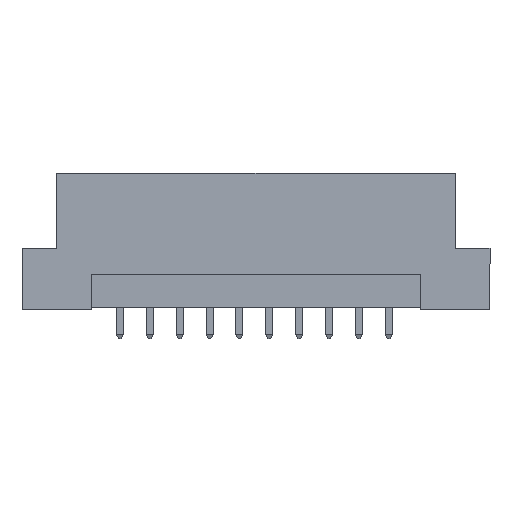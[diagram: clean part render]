
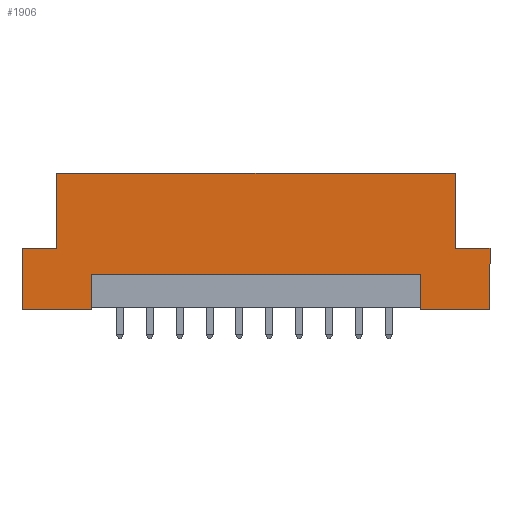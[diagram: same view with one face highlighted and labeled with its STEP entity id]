
A CAD part, front view. The second image highlights one B-rep face of the part: STEP entity #1906.
In plain terms, the highlighted planar face has unit normal (0, -1, 0).
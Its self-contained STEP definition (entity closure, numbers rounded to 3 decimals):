
#45 = VECTOR ( 'NONE', #1251, 1000. ) ;
#107 = ORIENTED_EDGE ( 'NONE', *, *, #4662, .T. ) ;
#114 = VERTEX_POINT ( 'NONE', #3270 ) ;
#131 = VECTOR ( 'NONE', #2270, 1000. ) ;
#250 = DIRECTION ( 'NONE',  ( 0., 0., 1. ) ) ;
#267 = EDGE_CURVE ( 'NONE', #1312, #3852, #4231, .T. ) ;
#430 = ORIENTED_EDGE ( 'NONE', *, *, #2387, .F. ) ;
#449 = CARTESIAN_POINT ( 'NONE',  ( -16.94, -4.3, 11.6 ) ) ;
#480 = VECTOR ( 'NONE', #901, 1000. ) ;
#522 = CARTESIAN_POINT ( 'NONE',  ( 19.9, -4.3, 0. ) ) ;
#525 = CARTESIAN_POINT ( 'NONE',  ( -14., -4.3, 3. ) ) ;
#536 = EDGE_CURVE ( 'NONE', #3905, #5048, #1664, .T. ) ;
#540 = LINE ( 'NONE', #2123, #2954 ) ;
#563 = ORIENTED_EDGE ( 'NONE', *, *, #3421, .F. ) ;
#606 = VECTOR ( 'NONE', #3008, 1000. ) ;
#608 = CARTESIAN_POINT ( 'NONE',  ( 19.9, -4.3, 11.6 ) ) ;
#617 = AXIS2_PLACEMENT_3D ( 'NONE', #4245, #5108, #2375 ) ;
#634 = CARTESIAN_POINT ( 'NONE',  ( -19.9, -4.3, 11.6 ) ) ;
#669 = EDGE_CURVE ( 'NONE', #3649, #3989, #4621, .T. ) ;
#682 = DIRECTION ( 'NONE',  ( 1., 0., 0. ) ) ;
#714 = CARTESIAN_POINT ( 'NONE',  ( -14., -4.3, 3. ) ) ;
#736 = VECTOR ( 'NONE', #1278, 1000. ) ;
#776 = VECTOR ( 'NONE', #1803, 1000. ) ;
#848 = VECTOR ( 'NONE', #2106, 1000. ) ;
#901 = DIRECTION ( 'NONE',  ( 0., 0., -1. ) ) ;
#1011 = LINE ( 'NONE', #1724, #776 ) ;
#1024 = VERTEX_POINT ( 'NONE', #3945 ) ;
#1050 = CARTESIAN_POINT ( 'NONE',  ( 19.9, -4.3, 0. ) ) ;
#1079 = DIRECTION ( 'NONE',  ( 1., 0., 0. ) ) ;
#1243 = EDGE_CURVE ( 'NONE', #3649, #114, #1011, .T. ) ;
#1251 = DIRECTION ( 'NONE',  ( 1., 0., 0. ) ) ;
#1278 = DIRECTION ( 'NONE',  ( 0., 0., -1. ) ) ;
#1280 = LINE ( 'NONE', #4136, #45 ) ;
#1312 = VERTEX_POINT ( 'NONE', #2902 ) ;
#1359 = VERTEX_POINT ( 'NONE', #525 ) ;
#1464 = CARTESIAN_POINT ( 'NONE',  ( -19.9, -4.3, 0. ) ) ;
#1664 = LINE ( 'NONE', #522, #848 ) ;
#1724 = CARTESIAN_POINT ( 'NONE',  ( 19.9, -4.3, 5.2 ) ) ;
#1803 = DIRECTION ( 'NONE',  ( 1., 0., 0. ) ) ;
#1861 = EDGE_LOOP ( 'NONE', ( #4857, #430, #3072, #4457, #3243, #2994, #4150, #563, #2382, #107, #2031, #2357 ) ) ;
#1906 = ADVANCED_FACE ( 'NONE', ( #3521 ), #3931, .F. ) ;
#1909 = CARTESIAN_POINT ( 'NONE',  ( 16.94, -4.3, 11.6 ) ) ;
#1931 = DIRECTION ( 'NONE',  ( 0., 0., -1. ) ) ;
#1942 = VECTOR ( 'NONE', #3540, 1000. ) ;
#2031 = ORIENTED_EDGE ( 'NONE', *, *, #536, .T. ) ;
#2106 = DIRECTION ( 'NONE',  ( 1., 0., 0. ) ) ;
#2123 = CARTESIAN_POINT ( 'NONE',  ( -16.94, -4.3, 5.2 ) ) ;
#2270 = DIRECTION ( 'NONE',  ( 1., 0., 0. ) ) ;
#2357 = ORIENTED_EDGE ( 'NONE', *, *, #4127, .F. ) ;
#2375 = DIRECTION ( 'NONE',  ( -1., 0., 0. ) ) ;
#2382 = ORIENTED_EDGE ( 'NONE', *, *, #3749, .F. ) ;
#2387 = EDGE_CURVE ( 'NONE', #1312, #3221, #2707, .T. ) ;
#2450 = EDGE_CURVE ( 'NONE', #2616, #3989, #4734, .T. ) ;
#2593 = VECTOR ( 'NONE', #682, 1000. ) ;
#2616 = VERTEX_POINT ( 'NONE', #449 ) ;
#2707 = LINE ( 'NONE', #3047, #1942 ) ;
#2868 = LINE ( 'NONE', #4453, #480 ) ;
#2902 = CARTESIAN_POINT ( 'NONE',  ( 14., -4.3, 0. ) ) ;
#2954 = VECTOR ( 'NONE', #250, 1000. ) ;
#2994 = ORIENTED_EDGE ( 'NONE', *, *, #669, .T. ) ;
#3008 = DIRECTION ( 'NONE',  ( 0., 0., 1. ) ) ;
#3047 = CARTESIAN_POINT ( 'NONE',  ( 14., -4.3, 0.2 ) ) ;
#3072 = ORIENTED_EDGE ( 'NONE', *, *, #267, .T. ) ;
#3204 = VERTEX_POINT ( 'NONE', #3625 ) ;
#3221 = VERTEX_POINT ( 'NONE', #4034 ) ;
#3243 = ORIENTED_EDGE ( 'NONE', *, *, #1243, .F. ) ;
#3270 = CARTESIAN_POINT ( 'NONE',  ( 19.9, -4.3, 5.2 ) ) ;
#3421 = EDGE_CURVE ( 'NONE', #1024, #2616, #540, .T. ) ;
#3426 = CARTESIAN_POINT ( 'NONE',  ( 16.94, -4.3, 5.2 ) ) ;
#3502 = CARTESIAN_POINT ( 'NONE',  ( -14., -4.3, 0. ) ) ;
#3521 = FACE_OUTER_BOUND ( 'NONE', #1861, .T. ) ;
#3540 = DIRECTION ( 'NONE',  ( 0., 0., 1. ) ) ;
#3625 = CARTESIAN_POINT ( 'NONE',  ( -19.9, -4.3, 5.2 ) ) ;
#3649 = VERTEX_POINT ( 'NONE', #4316 ) ;
#3749 = EDGE_CURVE ( 'NONE', #3204, #1024, #1280, .T. ) ;
#3832 = EDGE_CURVE ( 'NONE', #1359, #3221, #4944, .T. ) ;
#3852 = VERTEX_POINT ( 'NONE', #1050 ) ;
#3905 = VERTEX_POINT ( 'NONE', #1464 ) ;
#3928 = CARTESIAN_POINT ( 'NONE',  ( 19.9, -4.3, 11.6 ) ) ;
#3931 = PLANE ( 'NONE',  #617 ) ;
#3945 = CARTESIAN_POINT ( 'NONE',  ( -16.94, -4.3, 5.2 ) ) ;
#3989 = VERTEX_POINT ( 'NONE', #1909 ) ;
#4034 = CARTESIAN_POINT ( 'NONE',  ( 14., -4.3, 3. ) ) ;
#4044 = VECTOR ( 'NONE', #1931, 1000. ) ;
#4127 = EDGE_CURVE ( 'NONE', #1359, #5048, #2868, .T. ) ;
#4136 = CARTESIAN_POINT ( 'NONE',  ( -19.9, -4.3, 5.2 ) ) ;
#4150 = ORIENTED_EDGE ( 'NONE', *, *, #2450, .F. ) ;
#4158 = LINE ( 'NONE', #608, #736 ) ;
#4185 = LINE ( 'NONE', #634, #4044 ) ;
#4231 = LINE ( 'NONE', #5019, #2593 ) ;
#4245 = CARTESIAN_POINT ( 'NONE',  ( 19.9, -4.3, 11.6 ) ) ;
#4316 = CARTESIAN_POINT ( 'NONE',  ( 16.94, -4.3, 5.2 ) ) ;
#4332 = VECTOR ( 'NONE', #1079, 1000. ) ;
#4453 = CARTESIAN_POINT ( 'NONE',  ( -14., -4.3, 0.2 ) ) ;
#4457 = ORIENTED_EDGE ( 'NONE', *, *, #4529, .F. ) ;
#4529 = EDGE_CURVE ( 'NONE', #114, #3852, #4158, .T. ) ;
#4621 = LINE ( 'NONE', #3426, #606 ) ;
#4662 = EDGE_CURVE ( 'NONE', #3204, #3905, #4185, .T. ) ;
#4734 = LINE ( 'NONE', #3928, #4332 ) ;
#4857 = ORIENTED_EDGE ( 'NONE', *, *, #3832, .T. ) ;
#4944 = LINE ( 'NONE', #714, #131 ) ;
#5019 = CARTESIAN_POINT ( 'NONE',  ( 19.9, -4.3, 0. ) ) ;
#5048 = VERTEX_POINT ( 'NONE', #3502 ) ;
#5108 = DIRECTION ( 'NONE',  ( 0., 1., 0. ) ) ;
